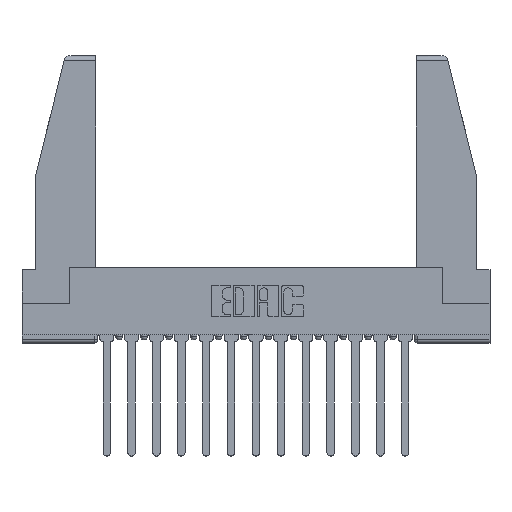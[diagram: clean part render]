
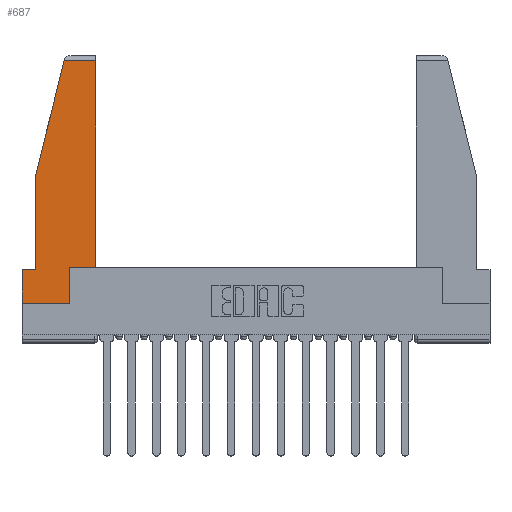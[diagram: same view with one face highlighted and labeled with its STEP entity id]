
A CAD part, top view. The second image highlights one B-rep face of the part: STEP entity #687.
In plain terms, the highlighted planar face has unit normal (0, 0, 1).
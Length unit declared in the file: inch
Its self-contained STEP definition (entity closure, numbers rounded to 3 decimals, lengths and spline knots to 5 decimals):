
#283 = CARTESIAN_POINT ( 'NONE',  ( 0.297, 0.223, 0. ) ) ;
#344 = VERTEX_POINT ( 'NONE', #15709 ) ;
#351 = CARTESIAN_POINT ( 'NONE',  ( 0.2636, 1.52, 0. ) ) ;
#616 = VECTOR ( 'NONE', #3516, 39.37008 ) ;
#687 = ADVANCED_FACE ( 'NONE', ( #3793 ), #4840, .T. ) ;
#723 = EDGE_CURVE ( 'NONE', #7971, #14243, #6496, .T. ) ;
#875 = DIRECTION ( 'NONE',  ( 1., 0., 0. ) ) ;
#1187 = DIRECTION ( 'NONE',  ( 1., 0., 0. ) ) ;
#1236 = EDGE_CURVE ( 'NONE', #344, #13691, #11697, .T. ) ;
#1244 = CARTESIAN_POINT ( 'NONE',  ( 0.086, 0.21, 0. ) ) ;
#1379 = EDGE_CURVE ( 'NONE', #13796, #2406, #8175, .T. ) ;
#1543 = CARTESIAN_POINT ( 'NONE',  ( 0., 0.21, 0. ) ) ;
#2197 = VECTOR ( 'NONE', #12815, 39.37008 ) ;
#2329 = ORIENTED_EDGE ( 'NONE', *, *, #16032, .T. ) ;
#2406 = VERTEX_POINT ( 'NONE', #14906 ) ;
#2813 = VECTOR ( 'NONE', #12306, 39.37008 ) ;
#2942 = LINE ( 'NONE', #4341, #4775 ) ;
#2995 = LINE ( 'NONE', #11180, #2813 ) ;
#3106 = DIRECTION ( 'NONE',  ( -1., 0., 0. ) ) ;
#3264 = LINE ( 'NONE', #8564, #616 ) ;
#3516 = DIRECTION ( 'NONE',  ( -0.239, -0.971, 0. ) ) ;
#3793 = FACE_OUTER_BOUND ( 'NONE', #5590, .T. ) ;
#4341 = CARTESIAN_POINT ( 'NONE',  ( 0., 0.21, 0. ) ) ;
#4497 = EDGE_CURVE ( 'NONE', #13691, #7177, #3264, .T. ) ;
#4775 = VECTOR ( 'NONE', #13637, 39.37008 ) ;
#4840 = PLANE ( 'NONE',  #7329 ) ;
#4979 = ORIENTED_EDGE ( 'NONE', *, *, #1236, .T. ) ;
#4987 = CARTESIAN_POINT ( 'NONE',  ( 0., 1.52, 0. ) ) ;
#5015 = CARTESIAN_POINT ( 'NONE',  ( 0., 0., 0. ) ) ;
#5287 = EDGE_CURVE ( 'NONE', #9739, #13796, #2942, .T. ) ;
#5565 = EDGE_CURVE ( 'NONE', #2406, #7971, #6419, .T. ) ;
#5590 = EDGE_LOOP ( 'NONE', ( #2329, #4979, #9797, #6916, #16760, #6507, #7922, #11764, #7454 ) ) ;
#6029 = CARTESIAN_POINT ( 'NONE',  ( 0.086, 0.8, 0. ) ) ;
#6215 = EDGE_CURVE ( 'NONE', #7177, #16262, #14092, .T. ) ;
#6419 = LINE ( 'NONE', #13109, #16146 ) ;
#6496 = LINE ( 'NONE', #15515, #8272 ) ;
#6507 = ORIENTED_EDGE ( 'NONE', *, *, #5287, .T. ) ;
#6916 = ORIENTED_EDGE ( 'NONE', *, *, #6215, .T. ) ;
#7177 = VERTEX_POINT ( 'NONE', #15762 ) ;
#7329 = AXIS2_PLACEMENT_3D ( 'NONE', #5015, #10325, #875 ) ;
#7454 = ORIENTED_EDGE ( 'NONE', *, *, #723, .T. ) ;
#7922 = ORIENTED_EDGE ( 'NONE', *, *, #1379, .T. ) ;
#7971 = VERTEX_POINT ( 'NONE', #283 ) ;
#8175 = LINE ( 'NONE', #9390, #13563 ) ;
#8272 = VECTOR ( 'NONE', #11719, 39.37008 ) ;
#8564 = CARTESIAN_POINT ( 'NONE',  ( 0.271, 1.55, 0. ) ) ;
#9390 = CARTESIAN_POINT ( 'NONE',  ( 0., 0., 0. ) ) ;
#9448 = CARTESIAN_POINT ( 'NONE',  ( 0., 0., 0. ) ) ;
#9739 = VERTEX_POINT ( 'NONE', #16309 ) ;
#9797 = ORIENTED_EDGE ( 'NONE', *, *, #4497, .T. ) ;
#10325 = DIRECTION ( 'NONE',  ( 0., 0., 1. ) ) ;
#10823 = CARTESIAN_POINT ( 'NONE',  ( 0.461, 0.223, 0. ) ) ;
#10896 = VECTOR ( 'NONE', #16368, 39.37008 ) ;
#11180 = CARTESIAN_POINT ( 'NONE',  ( 0.461, 0.223, 0. ) ) ;
#11697 = LINE ( 'NONE', #4987, #2197 ) ;
#11719 = DIRECTION ( 'NONE',  ( 1., 0., 0. ) ) ;
#11764 = ORIENTED_EDGE ( 'NONE', *, *, #5565, .T. ) ;
#12306 = DIRECTION ( 'NONE',  ( 0., 1., 0. ) ) ;
#12815 = DIRECTION ( 'NONE',  ( -1., 0., 0. ) ) ;
#13109 = CARTESIAN_POINT ( 'NONE',  ( 0.297, 0., 0. ) ) ;
#13518 = LINE ( 'NONE', #1543, #15277 ) ;
#13563 = VECTOR ( 'NONE', #1187, 39.37008 ) ;
#13637 = DIRECTION ( 'NONE',  ( 0., -1., 0. ) ) ;
#13691 = VERTEX_POINT ( 'NONE', #351 ) ;
#13796 = VERTEX_POINT ( 'NONE', #9448 ) ;
#14092 = LINE ( 'NONE', #6029, #10896 ) ;
#14243 = VERTEX_POINT ( 'NONE', #10823 ) ;
#14906 = CARTESIAN_POINT ( 'NONE',  ( 0.297, 0., 0. ) ) ;
#15106 = EDGE_CURVE ( 'NONE', #16262, #9739, #13518, .T. ) ;
#15277 = VECTOR ( 'NONE', #3106, 39.37008 ) ;
#15515 = CARTESIAN_POINT ( 'NONE',  ( 0.297, 0.223, 0. ) ) ;
#15709 = CARTESIAN_POINT ( 'NONE',  ( 0.461, 1.52, 0. ) ) ;
#15762 = CARTESIAN_POINT ( 'NONE',  ( 0.086, 0.8, 0. ) ) ;
#16032 = EDGE_CURVE ( 'NONE', #14243, #344, #2995, .T. ) ;
#16146 = VECTOR ( 'NONE', #17013, 39.37008 ) ;
#16262 = VERTEX_POINT ( 'NONE', #1244 ) ;
#16309 = CARTESIAN_POINT ( 'NONE',  ( 0., 0.21, 0. ) ) ;
#16368 = DIRECTION ( 'NONE',  ( 0., -1., 0. ) ) ;
#16760 = ORIENTED_EDGE ( 'NONE', *, *, #15106, .T. ) ;
#17013 = DIRECTION ( 'NONE',  ( 0., 1., 0. ) ) ;
